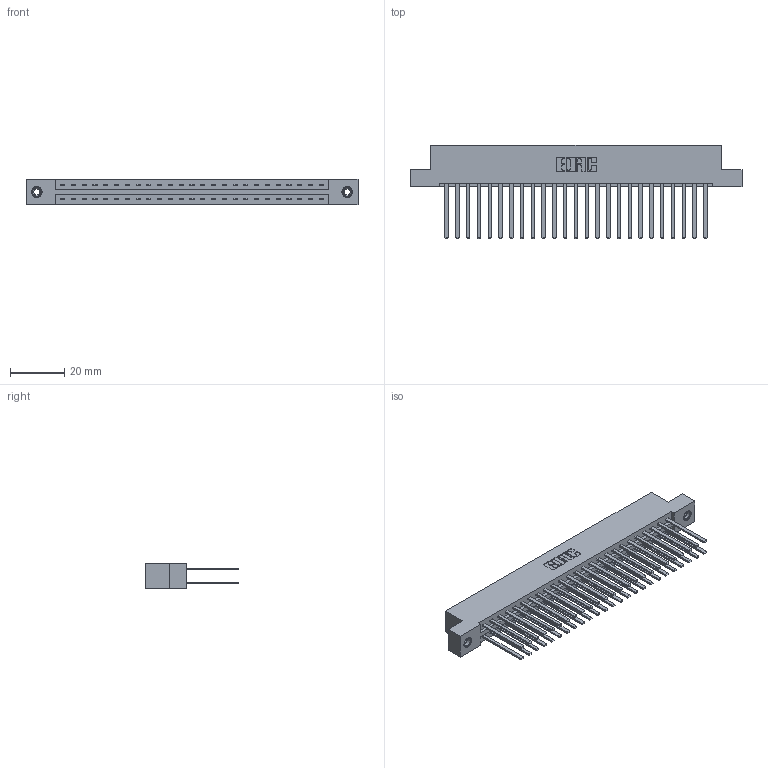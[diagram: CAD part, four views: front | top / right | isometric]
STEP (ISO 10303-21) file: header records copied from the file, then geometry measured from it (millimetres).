
FILE_DESCRIPTION (( 'STEP AP203' ), '1' );
FILE_NAME ('337-050-544-208.STEP', '2018-08-09T21:15:24', ( '' ), ( '' ), 'SwSTEP 2.0', 'SolidWorks 2016', '' );
FILE_SCHEMA (( 'CONFIG_CONTROL_DESIGN' ));
Length unit declared in the file: inch
Products named in the file (4): 345-250-001_345-250-003-102; 337-050-544-208; 337 Part_Flush Mounting Lugs - 0.156 Dia-TI; 345-292-001_345-293-144
Assembly tree (53 placements, depth 2):
  337-050-544-208
    337 Part_Flush Mounting Lugs - 0.156 Dia-TI
    345-292-001_345-293-144  x50
    345-250-001_345-250-003-102  x2
Bounding box: 122.07 x 34.3 x 9.4 mm (x, y, z)
Volume: 13333.1 mm3; surface area: 17221.5 mm2
Topology: 53 solids, 53 shells, 2574 faces, 7597 edges, 4990 vertices
Faces by surface type: plane 1802, cylinder 756, cone 12, torus 4
Entity records: 22584 total; most frequent: CARTESIAN_POINT 3797, ORIENTED_EDGE 3726, DIRECTION 3289, EDGE_CURVE 1863, VECTOR 1719, LINE 1719, VERTEX_POINT 1236, AXIS2_PLACEMENT_3D 785
